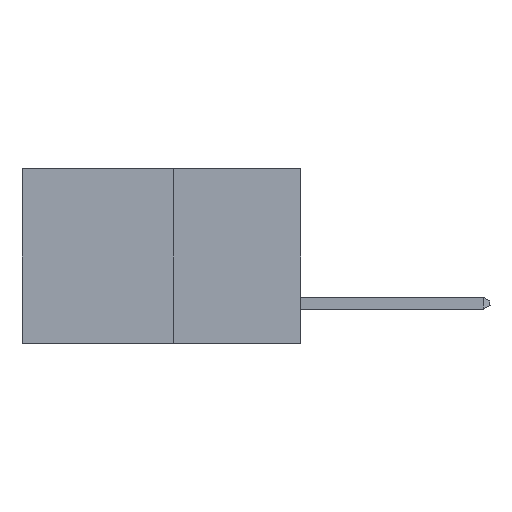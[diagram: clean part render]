
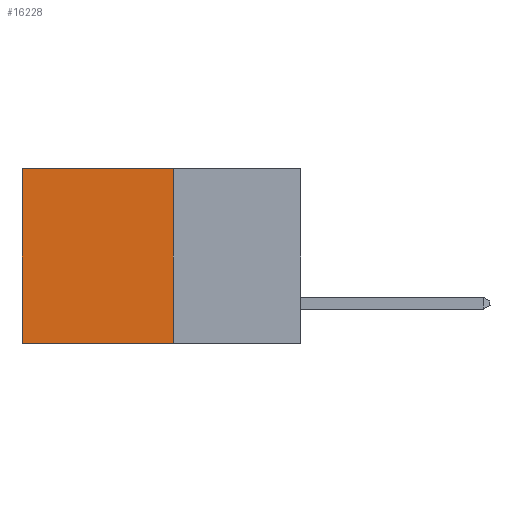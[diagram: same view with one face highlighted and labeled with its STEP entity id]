
A CAD part, left-side view. The second image highlights one B-rep face of the part: STEP entity #16228.
In plain terms, the highlighted planar face has unit normal (-1, 0, 0).
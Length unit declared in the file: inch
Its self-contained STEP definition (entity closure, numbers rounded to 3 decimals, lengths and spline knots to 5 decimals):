
#225 = DIRECTION ( 'NONE',  ( 0., 1., 0. ) ) ;
#567 = CARTESIAN_POINT ( 'NONE',  ( 0.277, 0.27, 0. ) ) ;
#1149 = LINE ( 'NONE', #9453, #12470 ) ;
#1819 = EDGE_CURVE ( 'NONE', #14502, #14466, #4520, .T. ) ;
#1925 = VECTOR ( 'NONE', #15207, 39.37008 ) ;
#2572 = ORIENTED_EDGE ( 'NONE', *, *, #7277, .T. ) ;
#2849 = CARTESIAN_POINT ( 'NONE',  ( 0.277, 0.27, -0.37 ) ) ;
#4051 = VECTOR ( 'NONE', #225, 39.37008 ) ;
#4086 = CARTESIAN_POINT ( 'NONE',  ( 0.277, 0.27, 0. ) ) ;
#4272 = ORIENTED_EDGE ( 'NONE', *, *, #1819, .F. ) ;
#4520 = LINE ( 'NONE', #16166, #4051 ) ;
#5894 = LINE ( 'NONE', #16590, #1925 ) ;
#5987 = LINE ( 'NONE', #4086, #13749 ) ;
#6738 = DIRECTION ( 'NONE',  ( 0., 1., 0. ) ) ;
#7093 = ORIENTED_EDGE ( 'NONE', *, *, #8526, .T. ) ;
#7239 = VERTEX_POINT ( 'NONE', #9942 ) ;
#7277 = EDGE_CURVE ( 'NONE', #7239, #14466, #1149, .T. ) ;
#8526 = EDGE_CURVE ( 'NONE', #8610, #7239, #5987, .T. ) ;
#8610 = VERTEX_POINT ( 'NONE', #567 ) ;
#8831 = DIRECTION ( 'NONE',  ( 1., 0., 0. ) ) ;
#9153 = FACE_OUTER_BOUND ( 'NONE', #17789, .T. ) ;
#9209 = ORIENTED_EDGE ( 'NONE', *, *, #10706, .F. ) ;
#9284 = AXIS2_PLACEMENT_3D ( 'NONE', #2849, #8831, #18958 ) ;
#9453 = CARTESIAN_POINT ( 'NONE',  ( 0.277, 0.59, -0.37 ) ) ;
#9762 = DIRECTION ( 'NONE',  ( 0., 0., -1. ) ) ;
#9942 = CARTESIAN_POINT ( 'NONE',  ( 0.277, 0.59, 0. ) ) ;
#10706 = EDGE_CURVE ( 'NONE', #8610, #14502, #5894, .T. ) ;
#12470 = VECTOR ( 'NONE', #9762, 39.37008 ) ;
#13749 = VECTOR ( 'NONE', #6738, 39.37008 ) ;
#14466 = VERTEX_POINT ( 'NONE', #15676 ) ;
#14502 = VERTEX_POINT ( 'NONE', #18652 ) ;
#15207 = DIRECTION ( 'NONE',  ( 0., 0., -1. ) ) ;
#15676 = CARTESIAN_POINT ( 'NONE',  ( 0.277, 0.59, -0.37 ) ) ;
#16166 = CARTESIAN_POINT ( 'NONE',  ( 0.277, 0.27, -0.37 ) ) ;
#16228 = ADVANCED_FACE ( 'NONE', ( #9153 ), #17513, .F. ) ;
#16590 = CARTESIAN_POINT ( 'NONE',  ( 0.277, 0.27, -0.37 ) ) ;
#17513 = PLANE ( 'NONE',  #9284 ) ;
#17789 = EDGE_LOOP ( 'NONE', ( #2572, #4272, #9209, #7093 ) ) ;
#18652 = CARTESIAN_POINT ( 'NONE',  ( 0.277, 0.27, -0.37 ) ) ;
#18958 = DIRECTION ( 'NONE',  ( 0., 0., -1. ) ) ;
